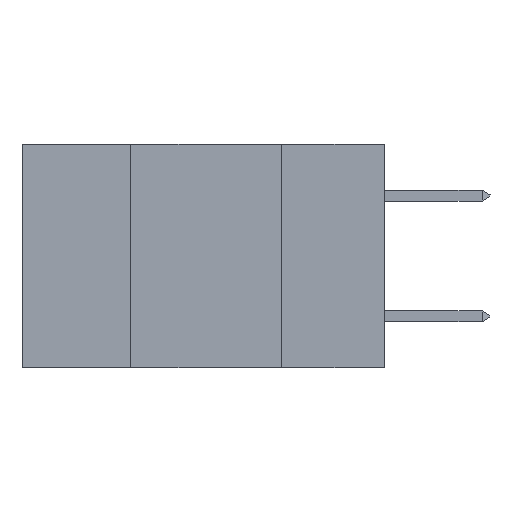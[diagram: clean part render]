
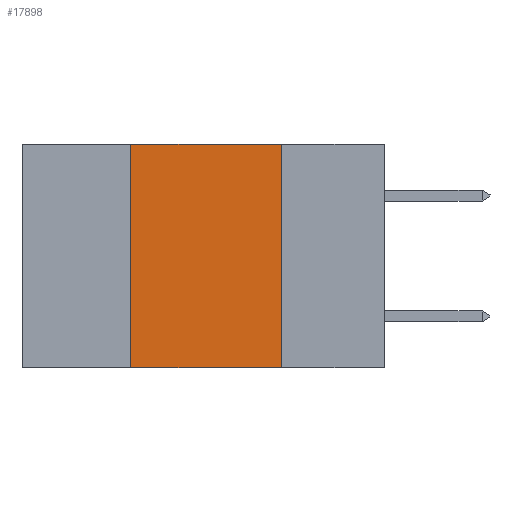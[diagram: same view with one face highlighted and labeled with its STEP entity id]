
A CAD part, left-side view. The second image highlights one B-rep face of the part: STEP entity #17898.
In plain terms, the highlighted planar face has unit normal (-1, 0, 0).
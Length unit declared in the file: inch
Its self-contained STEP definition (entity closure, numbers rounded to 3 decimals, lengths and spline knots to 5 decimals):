
#2751 = CARTESIAN_POINT ( 'NONE',  ( 0., 0.6, 0. ) ) ;
#3357 = CARTESIAN_POINT ( 'NONE',  ( 0., 0.17, 0. ) ) ;
#4097 = CARTESIAN_POINT ( 'NONE',  ( 0., 0.6, -0.37 ) ) ;
#4490 = DIRECTION ( 'NONE',  ( 0., 0., -1. ) ) ;
#6266 = ORIENTED_EDGE ( 'NONE', *, *, #31633, .F. ) ;
#8913 = DIRECTION ( 'NONE',  ( 1., 0., 0. ) ) ;
#9626 = VECTOR ( 'NONE', #4490, 39.37008 ) ;
#9646 = CARTESIAN_POINT ( 'NONE',  ( 0., 0.42, 0. ) ) ;
#10231 = LINE ( 'NONE', #9646, #18419 ) ;
#10957 = EDGE_LOOP ( 'NONE', ( #6266, #12638, #29494, #15269 ) ) ;
#12638 = ORIENTED_EDGE ( 'NONE', *, *, #17097, .F. ) ;
#13439 = PLANE ( 'NONE',  #28498 ) ;
#14329 = CARTESIAN_POINT ( 'NONE',  ( 0., 0.42, -0.37 ) ) ;
#15269 = ORIENTED_EDGE ( 'NONE', *, *, #17399, .T. ) ;
#15420 = CARTESIAN_POINT ( 'NONE',  ( 0., 0.17, -0.37 ) ) ;
#16800 = FACE_OUTER_BOUND ( 'NONE', #10957, .T. ) ;
#16825 = VECTOR ( 'NONE', #16827, 39.37008 ) ;
#16827 = DIRECTION ( 'NONE',  ( 0., -1., 0. ) ) ;
#17097 = EDGE_CURVE ( 'NONE', #31528, #26853, #31387, .T. ) ;
#17399 = EDGE_CURVE ( 'NONE', #17746, #26343, #29005, .T. ) ;
#17746 = VERTEX_POINT ( 'NONE', #14329 ) ;
#17898 = ADVANCED_FACE ( 'NONE', ( #16800 ), #13439, .F. ) ;
#18419 = VECTOR ( 'NONE', #27165, 39.37008 ) ;
#19216 = CARTESIAN_POINT ( 'NONE',  ( 0., 0.17, 0. ) ) ;
#19225 = VECTOR ( 'NONE', #28002, 39.37008 ) ;
#23681 = DIRECTION ( 'NONE',  ( 0., 0., -1. ) ) ;
#24496 = LINE ( 'NONE', #19216, #9626 ) ;
#25006 = EDGE_CURVE ( 'NONE', #17746, #31528, #10231, .T. ) ;
#26343 = VERTEX_POINT ( 'NONE', #15420 ) ;
#26853 = VERTEX_POINT ( 'NONE', #3357 ) ;
#27165 = DIRECTION ( 'NONE',  ( 0., 0., 1. ) ) ;
#28002 = DIRECTION ( 'NONE',  ( 0., -1., 0. ) ) ;
#28498 = AXIS2_PLACEMENT_3D ( 'NONE', #29184, #8913, #23681 ) ;
#28870 = CARTESIAN_POINT ( 'NONE',  ( 0., 0.42, 0. ) ) ;
#29005 = LINE ( 'NONE', #4097, #16825 ) ;
#29184 = CARTESIAN_POINT ( 'NONE',  ( 0., 0.6, 0. ) ) ;
#29494 = ORIENTED_EDGE ( 'NONE', *, *, #25006, .F. ) ;
#31387 = LINE ( 'NONE', #2751, #19225 ) ;
#31528 = VERTEX_POINT ( 'NONE', #28870 ) ;
#31633 = EDGE_CURVE ( 'NONE', #26853, #26343, #24496, .T. ) ;
